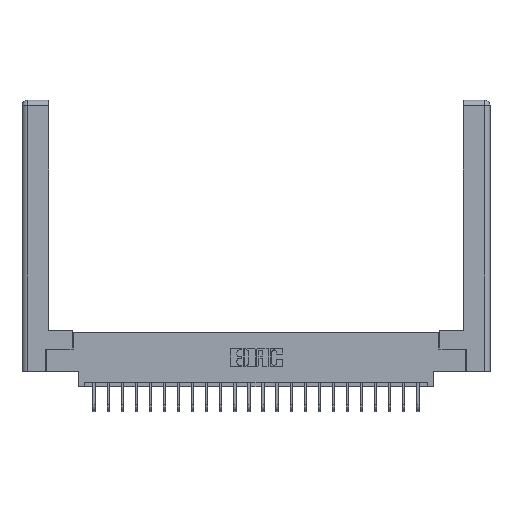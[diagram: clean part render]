
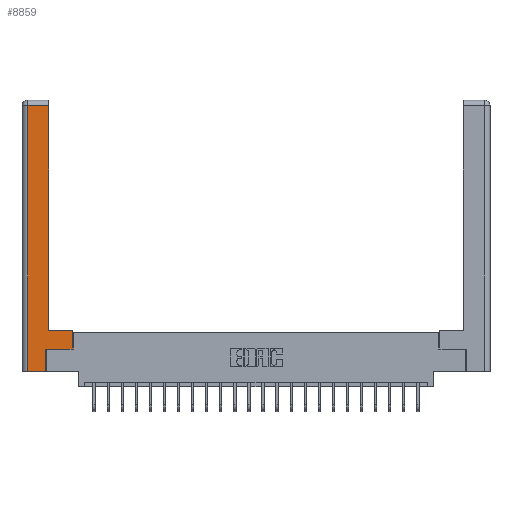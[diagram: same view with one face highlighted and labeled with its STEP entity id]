
A CAD part, top view. The second image highlights one B-rep face of the part: STEP entity #8859.
In plain terms, the highlighted planar face has unit normal (0, 0, 1).
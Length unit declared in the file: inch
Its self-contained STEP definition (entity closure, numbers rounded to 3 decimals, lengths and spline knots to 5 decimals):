
#38 = CARTESIAN_POINT ( 'NONE',  ( 0.265, 0., 0. ) ) ;
#467 = VECTOR ( 'NONE', #20458, 39.37008 ) ;
#521 = ORIENTED_EDGE ( 'NONE', *, *, #12621, .T. ) ;
#613 = DIRECTION ( 'NONE',  ( 0., 0., -1. ) ) ;
#1103 = EDGE_CURVE ( 'NONE', #12310, #15651, #21286, .T. ) ;
#1509 = ORIENTED_EDGE ( 'NONE', *, *, #15904, .T. ) ;
#1541 = VECTOR ( 'NONE', #10614, 39.37008 ) ;
#2489 = ORIENTED_EDGE ( 'NONE', *, *, #3347, .T. ) ;
#3347 = EDGE_CURVE ( 'NONE', #13216, #14097, #14900, .T. ) ;
#3521 = CARTESIAN_POINT ( 'NONE',  ( 0.265, 0.245, 0. ) ) ;
#4815 = ORIENTED_EDGE ( 'NONE', *, *, #7547, .T. ) ;
#4926 = VECTOR ( 'NONE', #8665, 39.37008 ) ;
#5719 = EDGE_LOOP ( 'NONE', ( #521, #12528, #10620, #11389, #4815, #16695, #1509, #2489 ) ) ;
#5964 = DIRECTION ( 'NONE',  ( -1., 0., 0. ) ) ;
#7481 = VERTEX_POINT ( 'NONE', #13508 ) ;
#7547 = EDGE_CURVE ( 'NONE', #7481, #21708, #9267, .T. ) ;
#7917 = CARTESIAN_POINT ( 'NONE',  ( 0., 0., 0. ) ) ;
#8222 = CARTESIAN_POINT ( 'NONE',  ( 0.565, 0.245, 0. ) ) ;
#8665 = DIRECTION ( 'NONE',  ( -1., 0., 0. ) ) ;
#8859 = ADVANCED_FACE ( 'NONE', ( #21065 ), #13328, .F. ) ;
#9203 = CARTESIAN_POINT ( 'NONE',  ( 0.265, 0.245, 0. ) ) ;
#9267 = LINE ( 'NONE', #9203, #12599 ) ;
#10614 = DIRECTION ( 'NONE',  ( 0., -1., 0. ) ) ;
#10620 = ORIENTED_EDGE ( 'NONE', *, *, #1103, .T. ) ;
#10844 = CARTESIAN_POINT ( 'NONE',  ( 0.0615, 0., 0. ) ) ;
#10854 = DIRECTION ( 'NONE',  ( 1., 0., 0. ) ) ;
#11103 = LINE ( 'NONE', #22256, #13913 ) ;
#11389 = ORIENTED_EDGE ( 'NONE', *, *, #15236, .T. ) ;
#11595 = CARTESIAN_POINT ( 'NONE',  ( 0.0615, 2.94, 0. ) ) ;
#12168 = VECTOR ( 'NONE', #18412, 39.37008 ) ;
#12310 = VERTEX_POINT ( 'NONE', #11595 ) ;
#12474 = VECTOR ( 'NONE', #10854, 39.37008 ) ;
#12528 = ORIENTED_EDGE ( 'NONE', *, *, #20684, .T. ) ;
#12599 = VECTOR ( 'NONE', #21549, 39.37008 ) ;
#12621 = EDGE_CURVE ( 'NONE', #14097, #19275, #21928, .T. ) ;
#13216 = VERTEX_POINT ( 'NONE', #20129 ) ;
#13328 = PLANE ( 'NONE',  #19470 ) ;
#13452 = EDGE_CURVE ( 'NONE', #21708, #21959, #17424, .T. ) ;
#13508 = CARTESIAN_POINT ( 'NONE',  ( 0.265, 0., 0. ) ) ;
#13913 = VECTOR ( 'NONE', #5964, 39.37008 ) ;
#14097 = VERTEX_POINT ( 'NONE', #17822 ) ;
#14110 = LINE ( 'NONE', #16469, #12168 ) ;
#14900 = LINE ( 'NONE', #17753, #4926 ) ;
#15236 = EDGE_CURVE ( 'NONE', #15651, #7481, #21425, .T. ) ;
#15514 = CARTESIAN_POINT ( 'NONE',  ( 0.295, 3., 0. ) ) ;
#15651 = VERTEX_POINT ( 'NONE', #19584 ) ;
#15904 = EDGE_CURVE ( 'NONE', #21959, #13216, #14110, .T. ) ;
#16469 = CARTESIAN_POINT ( 'NONE',  ( 0.565, 0.45, 0. ) ) ;
#16695 = ORIENTED_EDGE ( 'NONE', *, *, #13452, .T. ) ;
#17172 = VECTOR ( 'NONE', #17220, 39.37008 ) ;
#17220 = DIRECTION ( 'NONE',  ( 0., 1., 0. ) ) ;
#17418 = CARTESIAN_POINT ( 'NONE',  ( 0.295, 2.94, 0. ) ) ;
#17424 = LINE ( 'NONE', #8222, #467 ) ;
#17753 = CARTESIAN_POINT ( 'NONE',  ( 0.295, 0.45, 0. ) ) ;
#17822 = CARTESIAN_POINT ( 'NONE',  ( 0.295, 0.45, 0. ) ) ;
#18412 = DIRECTION ( 'NONE',  ( 0., 1., 0. ) ) ;
#19275 = VERTEX_POINT ( 'NONE', #17418 ) ;
#19470 = AXIS2_PLACEMENT_3D ( 'NONE', #7917, #613, #20277 ) ;
#19584 = CARTESIAN_POINT ( 'NONE',  ( 0.0615, 0., 0. ) ) ;
#20129 = CARTESIAN_POINT ( 'NONE',  ( 0.565, 0.45, 0. ) ) ;
#20197 = CARTESIAN_POINT ( 'NONE',  ( 0.565, 0.245, 0. ) ) ;
#20277 = DIRECTION ( 'NONE',  ( -1., 0., 0. ) ) ;
#20458 = DIRECTION ( 'NONE',  ( 1., 0., 0. ) ) ;
#20684 = EDGE_CURVE ( 'NONE', #19275, #12310, #11103, .T. ) ;
#21065 = FACE_OUTER_BOUND ( 'NONE', #5719, .T. ) ;
#21286 = LINE ( 'NONE', #10844, #1541 ) ;
#21425 = LINE ( 'NONE', #38, #12474 ) ;
#21549 = DIRECTION ( 'NONE',  ( 0., 1., 0. ) ) ;
#21708 = VERTEX_POINT ( 'NONE', #3521 ) ;
#21928 = LINE ( 'NONE', #15514, #17172 ) ;
#21959 = VERTEX_POINT ( 'NONE', #20197 ) ;
#22256 = CARTESIAN_POINT ( 'NONE',  ( 0.0615, 2.94, 0. ) ) ;
